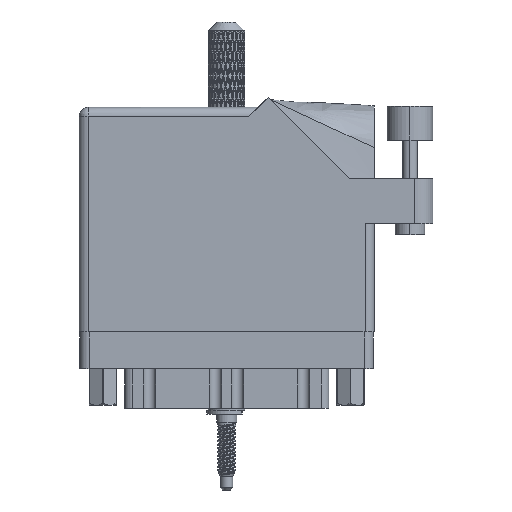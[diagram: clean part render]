
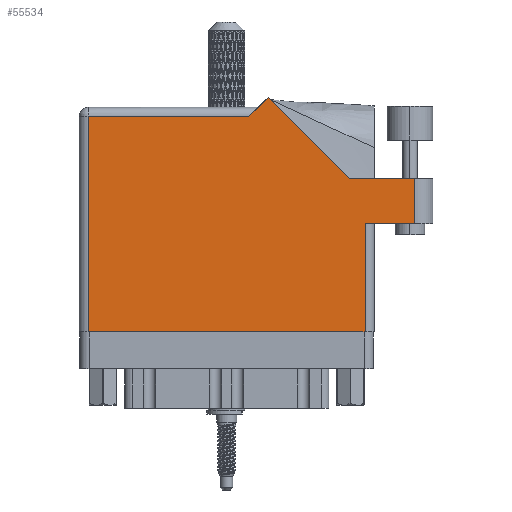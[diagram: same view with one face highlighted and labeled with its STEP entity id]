
A CAD part, front view. The second image highlights one B-rep face of the part: STEP entity #55534.
In plain terms, the highlighted face is planar.
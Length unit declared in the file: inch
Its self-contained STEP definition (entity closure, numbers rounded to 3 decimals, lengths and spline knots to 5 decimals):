
#789 = VECTOR ( 'NONE', #101938, 39.37008 ) ;
#1533 = CARTESIAN_POINT ( 'NONE',  ( 2.41, 1.044, 0. ) ) ;
#2253 = EDGE_CURVE ( 'NONE', #58280, #10329, #13421, .T. ) ;
#3612 = CARTESIAN_POINT ( 'NONE',  ( 2.01, 0.737, 0. ) ) ;
#4210 = CARTESIAN_POINT ( 'NONE',  ( 0., 1.53, 0. ) ) ;
#6206 = VECTOR ( 'NONE', #42247, 39.37008 ) ;
#6742 = CARTESIAN_POINT ( 'NONE',  ( 2.285, 0.737, 0. ) ) ;
#7807 = EDGE_CURVE ( 'NONE', #70042, #86507, #16091, .T. ) ;
#10329 = VERTEX_POINT ( 'NONE', #52865 ) ;
#11356 = ORIENTED_EDGE ( 'NONE', *, *, #32654, .T. ) ;
#12611 = EDGE_CURVE ( 'NONE', #70570, #71832, #61955, .T. ) ;
#13421 = LINE ( 'NONE', #84384, #111182 ) ;
#16091 = LINE ( 'NONE', #49303, #22070 ) ;
#16363 = CARTESIAN_POINT ( 'NONE',  ( 1.84442, 1.044, 0. ) ) ;
#16496 = CARTESIAN_POINT ( 'NONE',  ( 0., 1.468, 0. ) ) ;
#16542 = DIRECTION ( 'NONE',  ( 0., -1., 0. ) ) ;
#16828 = ORIENTED_EDGE ( 'NONE', *, *, #12611, .T. ) ;
#18220 = LINE ( 'NONE', #25115, #63158 ) ;
#21270 = CARTESIAN_POINT ( 'NONE',  ( 1.28771, 1.60071, 0. ) ) ;
#21397 = ORIENTED_EDGE ( 'NONE', *, *, #2253, .T. ) ;
#22070 = VECTOR ( 'NONE', #40676, 39.37008 ) ;
#25115 = CARTESIAN_POINT ( 'NONE',  ( 0.062, 0., 0. ) ) ;
#27369 = ORIENTED_EDGE ( 'NONE', *, *, #32718, .T. ) ;
#28577 = EDGE_CURVE ( 'NONE', #91581, #100750, #18220, .T. ) ;
#30070 = CARTESIAN_POINT ( 'NONE',  ( 1.155, 1.468, 0. ) ) ;
#31598 = CARTESIAN_POINT ( 'NONE',  ( 0., 0., 0. ) ) ;
#31634 = FACE_OUTER_BOUND ( 'NONE', #33406, .T. ) ;
#32654 = EDGE_CURVE ( 'NONE', #10329, #70570, #82053, .T. ) ;
#32718 = EDGE_CURVE ( 'NONE', #100750, #58280, #48239, .T. ) ;
#33406 = EDGE_LOOP ( 'NONE', ( #11356, #16828, #72021, #113125, #65258, #97325, #50243, #27369, #21397 ) ) ;
#40676 = DIRECTION ( 'NONE',  ( -0.707, -0.707, 0. ) ) ;
#42079 = CARTESIAN_POINT ( 'NONE',  ( 0.062, 1.468, 0. ) ) ;
#42247 = DIRECTION ( 'NONE',  ( -1., 0., 0. ) ) ;
#46832 = CARTESIAN_POINT ( 'NONE',  ( 1.84442, 1.044, 0. ) ) ;
#48239 = LINE ( 'NONE', #31598, #70333 ) ;
#49303 = CARTESIAN_POINT ( 'NONE',  ( 1.217, 1.53, 0. ) ) ;
#50243 = ORIENTED_EDGE ( 'NONE', *, *, #28577, .T. ) ;
#50389 = CARTESIAN_POINT ( 'NONE',  ( 1.948, 0., 0. ) ) ;
#52865 = CARTESIAN_POINT ( 'NONE',  ( 1.948, 0.737, 0. ) ) ;
#55534 = ADVANCED_FACE ( 'NONE', ( #31634 ), #82659, .F. ) ;
#56852 = DIRECTION ( 'NONE',  ( 1., 0., 0. ) ) ;
#58280 = VERTEX_POINT ( 'NONE', #50389 ) ;
#59602 = LINE ( 'NONE', #1533, #789 ) ;
#61955 = LINE ( 'NONE', #96842, #83098 ) ;
#63158 = VECTOR ( 'NONE', #16542, 39.37008 ) ;
#65258 = ORIENTED_EDGE ( 'NONE', *, *, #7807, .T. ) ;
#65699 = LINE ( 'NONE', #46832, #66856 ) ;
#66220 = AXIS2_PLACEMENT_3D ( 'NONE', #4210, #100900, #66559 ) ;
#66559 = DIRECTION ( 'NONE',  ( -1., 0., 0. ) ) ;
#66856 = VECTOR ( 'NONE', #108083, 39.37008 ) ;
#67428 = CARTESIAN_POINT ( 'NONE',  ( 0.062, 0., 0. ) ) ;
#69968 = DIRECTION ( 'NONE',  ( 0., 1., 0. ) ) ;
#70042 = VERTEX_POINT ( 'NONE', #21270 ) ;
#70333 = VECTOR ( 'NONE', #56852, 39.37008 ) ;
#70570 = VERTEX_POINT ( 'NONE', #6742 ) ;
#71832 = VERTEX_POINT ( 'NONE', #96567 ) ;
#72021 = ORIENTED_EDGE ( 'NONE', *, *, #102896, .T. ) ;
#72120 = VERTEX_POINT ( 'NONE', #16363 ) ;
#78293 = LINE ( 'NONE', #16496, #6206 ) ;
#82053 = LINE ( 'NONE', #3612, #103161 ) ;
#82659 = PLANE ( 'NONE',  #66220 ) ;
#83098 = VECTOR ( 'NONE', #69968, 39.37008 ) ;
#83179 = DIRECTION ( 'NONE',  ( 1., 0., 0. ) ) ;
#84384 = CARTESIAN_POINT ( 'NONE',  ( 1.948, 0.737, 0. ) ) ;
#86507 = VERTEX_POINT ( 'NONE', #30070 ) ;
#91581 = VERTEX_POINT ( 'NONE', #42079 ) ;
#91856 = DIRECTION ( 'NONE',  ( 0., 1., 0. ) ) ;
#96567 = CARTESIAN_POINT ( 'NONE',  ( 2.285, 1.044, 0. ) ) ;
#96842 = CARTESIAN_POINT ( 'NONE',  ( 2.285, 1.044, 0. ) ) ;
#97325 = ORIENTED_EDGE ( 'NONE', *, *, #101873, .T. ) ;
#100750 = VERTEX_POINT ( 'NONE', #67428 ) ;
#100900 = DIRECTION ( 'NONE',  ( 0., 0., -1. ) ) ;
#101873 = EDGE_CURVE ( 'NONE', #86507, #91581, #78293, .T. ) ;
#101938 = DIRECTION ( 'NONE',  ( -1., 0., 0. ) ) ;
#102896 = EDGE_CURVE ( 'NONE', #71832, #72120, #59602, .T. ) ;
#103161 = VECTOR ( 'NONE', #83179, 39.37008 ) ;
#105817 = EDGE_CURVE ( 'NONE', #72120, #70042, #65699, .T. ) ;
#108083 = DIRECTION ( 'NONE',  ( -0.707, 0.707, 0. ) ) ;
#111182 = VECTOR ( 'NONE', #91856, 39.37008 ) ;
#113125 = ORIENTED_EDGE ( 'NONE', *, *, #105817, .T. ) ;
